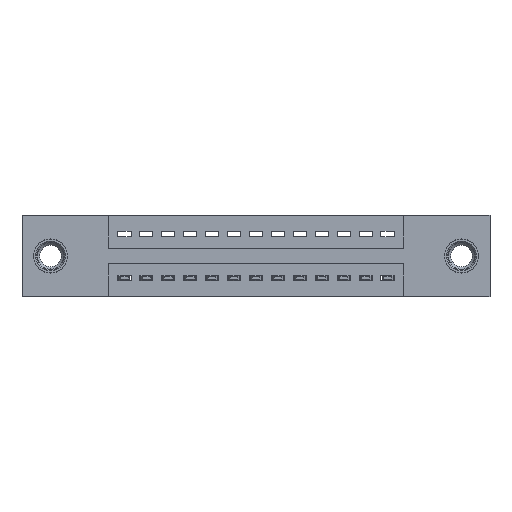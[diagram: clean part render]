
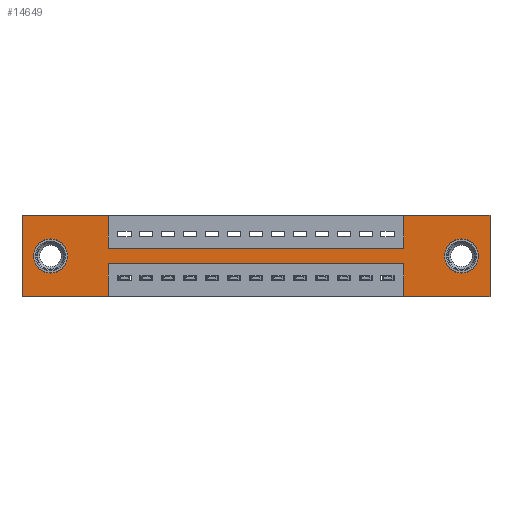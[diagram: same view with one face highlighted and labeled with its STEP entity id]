
A CAD part, front view. The second image highlights one B-rep face of the part: STEP entity #14649.
In plain terms, the highlighted planar face has unit normal (0, -1, 0).
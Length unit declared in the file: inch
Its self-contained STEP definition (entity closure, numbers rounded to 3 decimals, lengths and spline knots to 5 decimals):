
#89 = CARTESIAN_POINT ( 'NONE',  ( 0., 0., 0. ) ) ;
#269 = VECTOR ( 'NONE', #12693, 39.37008 ) ;
#278 = DIRECTION ( 'NONE',  ( 0., 1., 0. ) ) ;
#311 = EDGE_CURVE ( 'NONE', #4824, #9343, #10912, .T. ) ;
#428 = VECTOR ( 'NONE', #2979, 39.37008 ) ;
#438 = VERTEX_POINT ( 'NONE', #14279 ) ;
#509 = CARTESIAN_POINT ( 'NONE',  ( 2.135, 0., -0.37 ) ) ;
#541 = CIRCLE ( 'NONE', #6715, 0.078 ) ;
#597 = CARTESIAN_POINT ( 'NONE',  ( 1.7425, 0., 0. ) ) ;
#628 = DIRECTION ( 'NONE',  ( 0., 0., -1. ) ) ;
#649 = VERTEX_POINT ( 'NONE', #10032 ) ;
#803 = ORIENTED_EDGE ( 'NONE', *, *, #6677, .F. ) ;
#815 = CARTESIAN_POINT ( 'NONE',  ( 0., 0., -0.37 ) ) ;
#884 = CARTESIAN_POINT ( 'NONE',  ( 2.135, 0., 0. ) ) ;
#914 = CARTESIAN_POINT ( 'NONE',  ( 0., 0., 0. ) ) ;
#964 = FACE_BOUND ( 'NONE', #1007, .T. ) ;
#1007 = EDGE_LOOP ( 'NONE', ( #10716, #4673 ) ) ;
#1053 = CIRCLE ( 'NONE', #12326, 0.078 ) ;
#1153 = LINE ( 'NONE', #914, #9135 ) ;
#1210 = LINE ( 'NONE', #1823, #9882 ) ;
#1271 = VECTOR ( 'NONE', #13411, 39.37008 ) ;
#1285 = VERTEX_POINT ( 'NONE', #11296 ) ;
#1331 = CARTESIAN_POINT ( 'NONE',  ( 1.7425, 0., -0.15 ) ) ;
#1620 = DIRECTION ( 'NONE',  ( 0., 1., 0. ) ) ;
#1823 = CARTESIAN_POINT ( 'NONE',  ( 2.135, 0., 0. ) ) ;
#1956 = EDGE_CURVE ( 'NONE', #12568, #3618, #13337, .T. ) ;
#2036 = CARTESIAN_POINT ( 'NONE',  ( 0., 0., -0.37 ) ) ;
#2058 = DIRECTION ( 'NONE',  ( 0., 0., -1. ) ) ;
#2091 = VERTEX_POINT ( 'NONE', #11714 ) ;
#2326 = VECTOR ( 'NONE', #7055, 39.37008 ) ;
#2344 = LINE ( 'NONE', #2036, #1271 ) ;
#2458 = ORIENTED_EDGE ( 'NONE', *, *, #11417, .F. ) ;
#2479 = CIRCLE ( 'NONE', #9119, 0.078 ) ;
#2692 = LINE ( 'NONE', #4876, #2326 ) ;
#2733 = AXIS2_PLACEMENT_3D ( 'NONE', #7416, #1620, #10863 ) ;
#2799 = DIRECTION ( 'NONE',  ( 0., 1., 0. ) ) ;
#2813 = ORIENTED_EDGE ( 'NONE', *, *, #311, .F. ) ;
#2856 = ORIENTED_EDGE ( 'NONE', *, *, #3990, .T. ) ;
#2979 = DIRECTION ( 'NONE',  ( 0., 0., -1. ) ) ;
#3513 = DIRECTION ( 'NONE',  ( 0., 0., -1. ) ) ;
#3618 = VERTEX_POINT ( 'NONE', #9739 ) ;
#3647 = EDGE_CURVE ( 'NONE', #4292, #3766, #13487, .T. ) ;
#3766 = VERTEX_POINT ( 'NONE', #884 ) ;
#3846 = LINE ( 'NONE', #11513, #269 ) ;
#3872 = ORIENTED_EDGE ( 'NONE', *, *, #12135, .F. ) ;
#3989 = VECTOR ( 'NONE', #5671, 39.37008 ) ;
#3990 = EDGE_CURVE ( 'NONE', #649, #13697, #541, .T. ) ;
#4144 = AXIS2_PLACEMENT_3D ( 'NONE', #815, #12188, #2058 ) ;
#4195 = DIRECTION ( 'NONE',  ( 0., 0., 1. ) ) ;
#4292 = VERTEX_POINT ( 'NONE', #597 ) ;
#4558 = VERTEX_POINT ( 'NONE', #11444 ) ;
#4673 = ORIENTED_EDGE ( 'NONE', *, *, #10214, .T. ) ;
#4752 = LINE ( 'NONE', #6845, #8802 ) ;
#4824 = VERTEX_POINT ( 'NONE', #14021 ) ;
#4876 = CARTESIAN_POINT ( 'NONE',  ( 1.7425, 0., -0.37 ) ) ;
#4901 = DIRECTION ( 'NONE',  ( -1., 0., 0. ) ) ;
#4923 = EDGE_LOOP ( 'NONE', ( #11796, #3872, #6389, #6273, #5174, #10650, #803, #2813, #2458, #9612, #8441, #7876 ) ) ;
#5063 = FACE_OUTER_BOUND ( 'NONE', #4923, .T. ) ;
#5174 = ORIENTED_EDGE ( 'NONE', *, *, #10571, .F. ) ;
#5192 = DIRECTION ( 'NONE',  ( 0., 0., -1. ) ) ;
#5349 = PLANE ( 'NONE',  #4144 ) ;
#5579 = EDGE_CURVE ( 'NONE', #13697, #649, #7583, .T. ) ;
#5671 = DIRECTION ( 'NONE',  ( 1., 0., 0. ) ) ;
#5745 = CARTESIAN_POINT ( 'NONE',  ( 2.005, 0., -0.185 ) ) ;
#5868 = VECTOR ( 'NONE', #4901, 39.37008 ) ;
#5961 = CARTESIAN_POINT ( 'NONE',  ( 0.3925, 0., -0.22 ) ) ;
#6273 = ORIENTED_EDGE ( 'NONE', *, *, #9158, .F. ) ;
#6299 = LINE ( 'NONE', #12110, #428 ) ;
#6389 = ORIENTED_EDGE ( 'NONE', *, *, #9480, .F. ) ;
#6677 = EDGE_CURVE ( 'NONE', #9343, #4292, #4752, .T. ) ;
#6715 = AXIS2_PLACEMENT_3D ( 'NONE', #7084, #278, #6943 ) ;
#6845 = CARTESIAN_POINT ( 'NONE',  ( 1.7425, 0., 0. ) ) ;
#6943 = DIRECTION ( 'NONE',  ( 0., 0., 1. ) ) ;
#7054 = VECTOR ( 'NONE', #12001, 39.37008 ) ;
#7055 = DIRECTION ( 'NONE',  ( 0., 0., 1. ) ) ;
#7084 = CARTESIAN_POINT ( 'NONE',  ( 0.13, 0., -0.185 ) ) ;
#7416 = CARTESIAN_POINT ( 'NONE',  ( 0.13, 0., -0.185 ) ) ;
#7583 = CIRCLE ( 'NONE', #2733, 0.078 ) ;
#7715 = EDGE_CURVE ( 'NONE', #4558, #14121, #6299, .T. ) ;
#7876 = ORIENTED_EDGE ( 'NONE', *, *, #14151, .F. ) ;
#8441 = ORIENTED_EDGE ( 'NONE', *, *, #14236, .F. ) ;
#8521 = CARTESIAN_POINT ( 'NONE',  ( 0., 0., -0.37 ) ) ;
#8539 = VECTOR ( 'NONE', #8757, 39.37008 ) ;
#8658 = LINE ( 'NONE', #12987, #12914 ) ;
#8757 = DIRECTION ( 'NONE',  ( 1., 0., 0. ) ) ;
#8802 = VECTOR ( 'NONE', #14690, 39.37008 ) ;
#9119 = AXIS2_PLACEMENT_3D ( 'NONE', #9572, #2799, #12890 ) ;
#9135 = VECTOR ( 'NONE', #4195, 39.37008 ) ;
#9158 = EDGE_CURVE ( 'NONE', #12712, #2091, #2344, .T. ) ;
#9191 = EDGE_LOOP ( 'NONE', ( #2856, #11149 ) ) ;
#9343 = VERTEX_POINT ( 'NONE', #1331 ) ;
#9480 = EDGE_CURVE ( 'NONE', #2091, #14242, #2692, .T. ) ;
#9572 = CARTESIAN_POINT ( 'NONE',  ( 2.005, 0., -0.185 ) ) ;
#9612 = ORIENTED_EDGE ( 'NONE', *, *, #1956, .F. ) ;
#9640 = FACE_BOUND ( 'NONE', #9191, .T. ) ;
#9739 = CARTESIAN_POINT ( 'NONE',  ( 0.3925, 0., 0. ) ) ;
#9746 = CARTESIAN_POINT ( 'NONE',  ( 0.3925, 0., -0.15 ) ) ;
#9882 = VECTOR ( 'NONE', #628, 39.37008 ) ;
#10032 = CARTESIAN_POINT ( 'NONE',  ( 0.13, 0., -0.107 ) ) ;
#10214 = EDGE_CURVE ( 'NONE', #1285, #438, #2479, .T. ) ;
#10571 = EDGE_CURVE ( 'NONE', #3766, #12712, #1210, .T. ) ;
#10650 = ORIENTED_EDGE ( 'NONE', *, *, #3647, .F. ) ;
#10662 = EDGE_CURVE ( 'NONE', #438, #1285, #1053, .T. ) ;
#10716 = ORIENTED_EDGE ( 'NONE', *, *, #10662, .T. ) ;
#10863 = DIRECTION ( 'NONE',  ( 0., 0., 1. ) ) ;
#10912 = LINE ( 'NONE', #9746, #7054 ) ;
#10916 = VERTEX_POINT ( 'NONE', #8521 ) ;
#11149 = ORIENTED_EDGE ( 'NONE', *, *, #5579, .T. ) ;
#11296 = CARTESIAN_POINT ( 'NONE',  ( 2.005, 0., -0.263 ) ) ;
#11297 = DIRECTION ( 'NONE',  ( 0., 1., 0. ) ) ;
#11417 = EDGE_CURVE ( 'NONE', #3618, #4824, #8658, .T. ) ;
#11444 = CARTESIAN_POINT ( 'NONE',  ( 0.3925, 0., -0.22 ) ) ;
#11513 = CARTESIAN_POINT ( 'NONE',  ( 0., 0., -0.37 ) ) ;
#11562 = CARTESIAN_POINT ( 'NONE',  ( 0.3925, 0., -0.37 ) ) ;
#11714 = CARTESIAN_POINT ( 'NONE',  ( 1.7425, 0., -0.37 ) ) ;
#11796 = ORIENTED_EDGE ( 'NONE', *, *, #7715, .F. ) ;
#11827 = LINE ( 'NONE', #5961, #5868 ) ;
#11876 = CARTESIAN_POINT ( 'NONE',  ( 0., 0., 0. ) ) ;
#12001 = DIRECTION ( 'NONE',  ( 1., 0., 0. ) ) ;
#12110 = CARTESIAN_POINT ( 'NONE',  ( 0.3925, 0., -0.37 ) ) ;
#12135 = EDGE_CURVE ( 'NONE', #14242, #4558, #11827, .T. ) ;
#12188 = DIRECTION ( 'NONE',  ( 0., -1., 0. ) ) ;
#12326 = AXIS2_PLACEMENT_3D ( 'NONE', #5745, #11297, #3513 ) ;
#12568 = VERTEX_POINT ( 'NONE', #11876 ) ;
#12693 = DIRECTION ( 'NONE',  ( -1., 0., 0. ) ) ;
#12712 = VERTEX_POINT ( 'NONE', #509 ) ;
#12890 = DIRECTION ( 'NONE',  ( 0., 0., -1. ) ) ;
#12914 = VECTOR ( 'NONE', #5192, 39.37008 ) ;
#12987 = CARTESIAN_POINT ( 'NONE',  ( 0.3925, 0., 0. ) ) ;
#13337 = LINE ( 'NONE', #89, #3989 ) ;
#13411 = DIRECTION ( 'NONE',  ( -1., 0., 0. ) ) ;
#13487 = LINE ( 'NONE', #14294, #8539 ) ;
#13697 = VERTEX_POINT ( 'NONE', #14714 ) ;
#14021 = CARTESIAN_POINT ( 'NONE',  ( 0.3925, 0., -0.15 ) ) ;
#14121 = VERTEX_POINT ( 'NONE', #11562 ) ;
#14151 = EDGE_CURVE ( 'NONE', #14121, #10916, #3846, .T. ) ;
#14236 = EDGE_CURVE ( 'NONE', #10916, #12568, #1153, .T. ) ;
#14242 = VERTEX_POINT ( 'NONE', #14424 ) ;
#14279 = CARTESIAN_POINT ( 'NONE',  ( 2.005, 0., -0.107 ) ) ;
#14294 = CARTESIAN_POINT ( 'NONE',  ( 0., 0., 0. ) ) ;
#14424 = CARTESIAN_POINT ( 'NONE',  ( 1.7425, 0., -0.22 ) ) ;
#14649 = ADVANCED_FACE ( 'NONE', ( #964, #9640, #5063 ), #5349, .T. ) ;
#14690 = DIRECTION ( 'NONE',  ( 0., 0., 1. ) ) ;
#14714 = CARTESIAN_POINT ( 'NONE',  ( 0.13, 0., -0.263 ) ) ;
